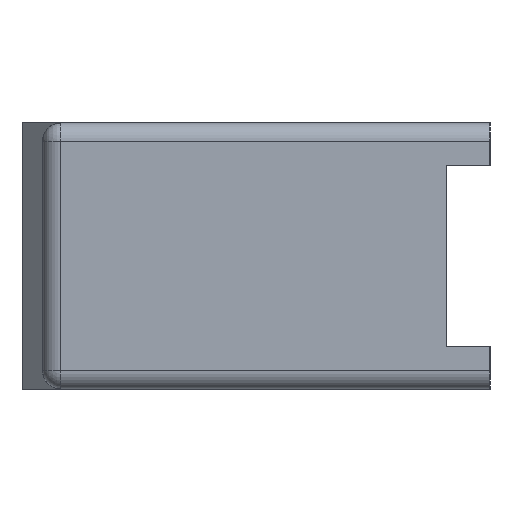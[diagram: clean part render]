
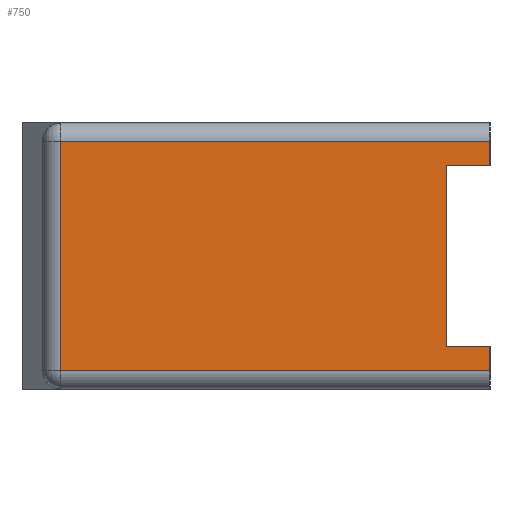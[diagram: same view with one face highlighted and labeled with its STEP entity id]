
A CAD part, left-side view. The second image highlights one B-rep face of the part: STEP entity #750.
In plain terms, the highlighted planar face has unit normal (-1, 0, 0).
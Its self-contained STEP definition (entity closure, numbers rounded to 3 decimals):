
#6 = ORIENTED_EDGE ( 'NONE', *, *, #1625, .T. ) ;
#20 = LINE ( 'NONE', #2334, #1850 ) ;
#102 = CARTESIAN_POINT ( 'NONE',  ( 0., 0., -23.114 ) ) ;
#107 = DIRECTION ( 'NONE',  ( 0., -1., 0. ) ) ;
#154 = EDGE_CURVE ( 'NONE', #253, #328, #1260, .T. ) ;
#183 = VERTEX_POINT ( 'NONE', #1186 ) ;
#216 = ORIENTED_EDGE ( 'NONE', *, *, #306, .T. ) ;
#244 = CARTESIAN_POINT ( 'NONE',  ( 0., 0., -21.539 ) ) ;
#253 = VERTEX_POINT ( 'NONE', #263 ) ;
#263 = CARTESIAN_POINT ( 'NONE',  ( 0., 0., -3.683 ) ) ;
#278 = ORIENTED_EDGE ( 'NONE', *, *, #154, .F. ) ;
#302 = DIRECTION ( 'NONE',  ( 0., 0., 1. ) ) ;
#306 = EDGE_CURVE ( 'NONE', #2362, #955, #1804, .T. ) ;
#314 = PLANE ( 'NONE',  #562 ) ;
#328 = VERTEX_POINT ( 'NONE', #1454 ) ;
#368 = CARTESIAN_POINT ( 'NONE',  ( 0., 0., -1.575 ) ) ;
#408 = DIRECTION ( 'NONE',  ( 0., 0., 1. ) ) ;
#418 = EDGE_CURVE ( 'NONE', #599, #183, #964, .T. ) ;
#526 = EDGE_CURVE ( 'NONE', #328, #1606, #20, .T. ) ;
#539 = VECTOR ( 'NONE', #577, 1000. ) ;
#562 = AXIS2_PLACEMENT_3D ( 'NONE', #102, #2437, #1997 ) ;
#577 = DIRECTION ( 'NONE',  ( 0., 0., -1. ) ) ;
#599 = VERTEX_POINT ( 'NONE', #368 ) ;
#630 = CARTESIAN_POINT ( 'NONE',  ( 0., 0., -19.431 ) ) ;
#664 = CARTESIAN_POINT ( 'NONE',  ( 0., 0., -23.114 ) ) ;
#750 = ADVANCED_FACE ( 'NONE', ( #882 ), #314, .T. ) ;
#815 = ORIENTED_EDGE ( 'NONE', *, *, #1566, .T. ) ;
#882 = FACE_OUTER_BOUND ( 'NONE', #1314, .T. ) ;
#937 = CARTESIAN_POINT ( 'NONE',  ( 0., 38.862, -1.575 ) ) ;
#955 = VERTEX_POINT ( 'NONE', #630 ) ;
#964 = LINE ( 'NONE', #937, #2504 ) ;
#985 = CARTESIAN_POINT ( 'NONE',  ( 0., 0., -23.114 ) ) ;
#994 = ORIENTED_EDGE ( 'NONE', *, *, #526, .F. ) ;
#1026 = DIRECTION ( 'NONE',  ( 0., 0., -1. ) ) ;
#1163 = CARTESIAN_POINT ( 'NONE',  ( 0., 3.81, -19.431 ) ) ;
#1183 = LINE ( 'NONE', #985, #1821 ) ;
#1186 = CARTESIAN_POINT ( 'NONE',  ( 0., 37.287, -1.575 ) ) ;
#1259 = CARTESIAN_POINT ( 'NONE',  ( 0., 0., -21.539 ) ) ;
#1260 = LINE ( 'NONE', #2371, #1903 ) ;
#1310 = EDGE_CURVE ( 'NONE', #1606, #955, #1469, .T. ) ;
#1314 = EDGE_LOOP ( 'NONE', ( #6, #2227, #216, #1464, #994, #278, #815, #1941 ) ) ;
#1425 = VECTOR ( 'NONE', #302, 1000. ) ;
#1441 = VERTEX_POINT ( 'NONE', #2471 ) ;
#1454 = CARTESIAN_POINT ( 'NONE',  ( 0., 3.81, -3.683 ) ) ;
#1464 = ORIENTED_EDGE ( 'NONE', *, *, #1310, .F. ) ;
#1469 = LINE ( 'NONE', #2244, #2120 ) ;
#1566 = EDGE_CURVE ( 'NONE', #253, #599, #1183, .T. ) ;
#1606 = VERTEX_POINT ( 'NONE', #1163 ) ;
#1608 = DIRECTION ( 'NONE',  ( 0., 1., 0. ) ) ;
#1625 = EDGE_CURVE ( 'NONE', #183, #1441, #2314, .T. ) ;
#1710 = DIRECTION ( 'NONE',  ( 0., 1., 0. ) ) ;
#1804 = LINE ( 'NONE', #664, #1425 ) ;
#1821 = VECTOR ( 'NONE', #408, 1000. ) ;
#1850 = VECTOR ( 'NONE', #1026, 1000. ) ;
#1903 = VECTOR ( 'NONE', #1608, 1000. ) ;
#1941 = ORIENTED_EDGE ( 'NONE', *, *, #418, .T. ) ;
#1948 = CARTESIAN_POINT ( 'NONE',  ( 0., 37.287, -23.114 ) ) ;
#1989 = VECTOR ( 'NONE', #2019, 1000. ) ;
#1997 = DIRECTION ( 'NONE',  ( 0., 0., 1. ) ) ;
#2019 = DIRECTION ( 'NONE',  ( 0., -1., 0. ) ) ;
#2084 = EDGE_CURVE ( 'NONE', #1441, #2362, #2366, .T. ) ;
#2120 = VECTOR ( 'NONE', #107, 1000. ) ;
#2227 = ORIENTED_EDGE ( 'NONE', *, *, #2084, .T. ) ;
#2244 = CARTESIAN_POINT ( 'NONE',  ( 0., 3.81, -19.431 ) ) ;
#2314 = LINE ( 'NONE', #1948, #539 ) ;
#2334 = CARTESIAN_POINT ( 'NONE',  ( 0., 3.81, -19.431 ) ) ;
#2362 = VERTEX_POINT ( 'NONE', #1259 ) ;
#2366 = LINE ( 'NONE', #244, #1989 ) ;
#2371 = CARTESIAN_POINT ( 'NONE',  ( 0., 3.81, -3.683 ) ) ;
#2437 = DIRECTION ( 'NONE',  ( -1., 0., 0. ) ) ;
#2471 = CARTESIAN_POINT ( 'NONE',  ( 0., 37.287, -21.539 ) ) ;
#2504 = VECTOR ( 'NONE', #1710, 1000. ) ;
